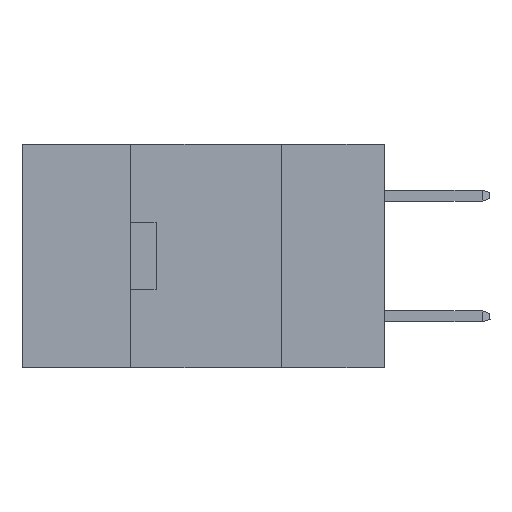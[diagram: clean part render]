
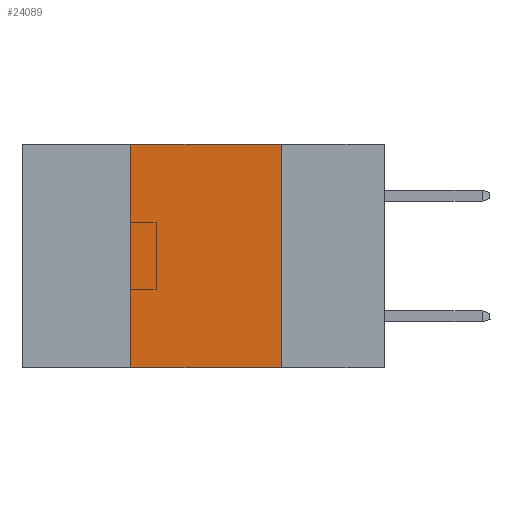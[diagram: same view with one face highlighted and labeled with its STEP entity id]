
A CAD part, left-side view. The second image highlights one B-rep face of the part: STEP entity #24089.
In plain terms, the highlighted planar face has unit normal (-1, 0, 0).
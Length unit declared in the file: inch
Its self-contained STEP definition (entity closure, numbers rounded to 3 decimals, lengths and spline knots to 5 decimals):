
#186 = CARTESIAN_POINT ( 'NONE',  ( 0., 0.42, 0. ) ) ;
#1241 = LINE ( 'NONE', #16559, #24321 ) ;
#4336 = ORIENTED_EDGE ( 'NONE', *, *, #16346, .F. ) ;
#4775 = DIRECTION ( 'NONE',  ( 0., 0., 1. ) ) ;
#7905 = CARTESIAN_POINT ( 'NONE',  ( 0., 0.17, 0. ) ) ;
#8412 = EDGE_CURVE ( 'NONE', #23980, #22565, #1241, .T. ) ;
#8726 = EDGE_LOOP ( 'NONE', ( #4336, #12121, #28882, #28571 ) ) ;
#9094 = CARTESIAN_POINT ( 'NONE',  ( 0., 0.17, -0.37 ) ) ;
#9510 = DIRECTION ( 'NONE',  ( 0., 0., -1. ) ) ;
#10324 = EDGE_CURVE ( 'NONE', #11699, #11290, #17426, .T. ) ;
#10868 = LINE ( 'NONE', #11611, #22599 ) ;
#11290 = VERTEX_POINT ( 'NONE', #7905 ) ;
#11611 = CARTESIAN_POINT ( 'NONE',  ( 0., 0.42, -0.37 ) ) ;
#11699 = VERTEX_POINT ( 'NONE', #186 ) ;
#12121 = ORIENTED_EDGE ( 'NONE', *, *, #10324, .F. ) ;
#13474 = VECTOR ( 'NONE', #24593, 39.37008 ) ;
#15203 = FACE_OUTER_BOUND ( 'NONE', #8726, .T. ) ;
#16346 = EDGE_CURVE ( 'NONE', #11290, #22565, #23757, .T. ) ;
#16559 = CARTESIAN_POINT ( 'NONE',  ( 0., 0.6, -0.37 ) ) ;
#16769 = AXIS2_PLACEMENT_3D ( 'NONE', #20547, #22754, #9510 ) ;
#17426 = LINE ( 'NONE', #19814, #22495 ) ;
#18377 = PLANE ( 'NONE',  #16769 ) ;
#19814 = CARTESIAN_POINT ( 'NONE',  ( 0., 0.6, 0. ) ) ;
#20182 = CARTESIAN_POINT ( 'NONE',  ( 0., 0.42, -0.37 ) ) ;
#20248 = CARTESIAN_POINT ( 'NONE',  ( 0., 0.17, -0.37 ) ) ;
#20323 = EDGE_CURVE ( 'NONE', #23980, #11699, #10868, .T. ) ;
#20547 = CARTESIAN_POINT ( 'NONE',  ( 0., 0.6, 0. ) ) ;
#22495 = VECTOR ( 'NONE', #26372, 39.37008 ) ;
#22565 = VERTEX_POINT ( 'NONE', #20248 ) ;
#22599 = VECTOR ( 'NONE', #4775, 39.37008 ) ;
#22754 = DIRECTION ( 'NONE',  ( 1., 0., 0. ) ) ;
#23757 = LINE ( 'NONE', #9094, #13474 ) ;
#23980 = VERTEX_POINT ( 'NONE', #20182 ) ;
#24089 = ADVANCED_FACE ( 'NONE', ( #15203 ), #18377, .F. ) ;
#24321 = VECTOR ( 'NONE', #25248, 39.37008 ) ;
#24593 = DIRECTION ( 'NONE',  ( 0., 0., -1. ) ) ;
#25248 = DIRECTION ( 'NONE',  ( 0., -1., 0. ) ) ;
#26372 = DIRECTION ( 'NONE',  ( 0., -1., 0. ) ) ;
#28571 = ORIENTED_EDGE ( 'NONE', *, *, #8412, .T. ) ;
#28882 = ORIENTED_EDGE ( 'NONE', *, *, #20323, .F. ) ;
